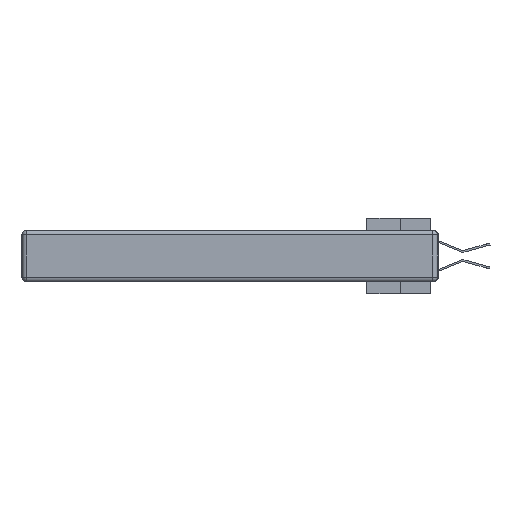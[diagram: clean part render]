
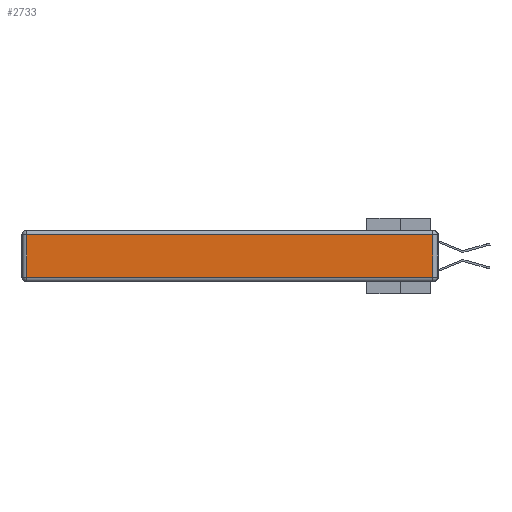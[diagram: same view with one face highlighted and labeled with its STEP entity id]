
A CAD part, left-side view. The second image highlights one B-rep face of the part: STEP entity #2733.
In plain terms, the highlighted planar face has unit normal (-1, 0, 0).
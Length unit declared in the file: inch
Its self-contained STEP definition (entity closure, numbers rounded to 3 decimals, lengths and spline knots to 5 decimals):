
#1680 = DIRECTION ( 'NONE',  ( 0., 0., -1. ) ) ;
#2733 = ADVANCED_FACE ( 'NONE', ( #30033 ), #18449, .T. ) ;
#3042 = CARTESIAN_POINT ( 'NONE',  ( 0., 0.03, -0.343 ) ) ;
#4611 = CARTESIAN_POINT ( 'NONE',  ( 0., 0., -0.343 ) ) ;
#4630 = CARTESIAN_POINT ( 'NONE',  ( 0., 0., -0.313 ) ) ;
#6864 = EDGE_CURVE ( 'NONE', #29253, #25889, #33131, .T. ) ;
#8099 = CARTESIAN_POINT ( 'NONE',  ( 0., 0.03, -0.313 ) ) ;
#9782 = DIRECTION ( 'NONE',  ( 0., -1., 0. ) ) ;
#9823 = VERTEX_POINT ( 'NONE', #8099 ) ;
#10138 = CARTESIAN_POINT ( 'NONE',  ( 0., 2.75, -0.03 ) ) ;
#11704 = AXIS2_PLACEMENT_3D ( 'NONE', #4611, #15663, #29659 ) ;
#13114 = CARTESIAN_POINT ( 'NONE',  ( 0., 2.72, -0.343 ) ) ;
#13416 = VECTOR ( 'NONE', #1680, 39.37008 ) ;
#14109 = EDGE_CURVE ( 'NONE', #9823, #29253, #22403, .T. ) ;
#15663 = DIRECTION ( 'NONE',  ( -1., 0., 0. ) ) ;
#18449 = PLANE ( 'NONE',  #11704 ) ;
#19187 = ORIENTED_EDGE ( 'NONE', *, *, #24821, .T. ) ;
#21542 = ORIENTED_EDGE ( 'NONE', *, *, #6864, .T. ) ;
#22403 = LINE ( 'NONE', #3042, #26266 ) ;
#22550 = VECTOR ( 'NONE', #35528, 39.37008 ) ;
#22754 = CARTESIAN_POINT ( 'NONE',  ( 0., 2.72, -0.03 ) ) ;
#24821 = EDGE_CURVE ( 'NONE', #30087, #9823, #34989, .T. ) ;
#25768 = ORIENTED_EDGE ( 'NONE', *, *, #14109, .T. ) ;
#25889 = VERTEX_POINT ( 'NONE', #22754 ) ;
#25919 = CARTESIAN_POINT ( 'NONE',  ( 0., 0.03, -0.03 ) ) ;
#25964 = CARTESIAN_POINT ( 'NONE',  ( 0., 2.72, -0.313 ) ) ;
#26266 = VECTOR ( 'NONE', #36200, 39.37008 ) ;
#26923 = LINE ( 'NONE', #13114, #13416 ) ;
#26992 = VECTOR ( 'NONE', #9782, 39.37008 ) ;
#28307 = ORIENTED_EDGE ( 'NONE', *, *, #34260, .T. ) ;
#29253 = VERTEX_POINT ( 'NONE', #25919 ) ;
#29659 = DIRECTION ( 'NONE',  ( 0., 0., 1. ) ) ;
#30033 = FACE_OUTER_BOUND ( 'NONE', #30587, .T. ) ;
#30087 = VERTEX_POINT ( 'NONE', #25964 ) ;
#30587 = EDGE_LOOP ( 'NONE', ( #19187, #25768, #21542, #28307 ) ) ;
#33131 = LINE ( 'NONE', #10138, #22550 ) ;
#34260 = EDGE_CURVE ( 'NONE', #25889, #30087, #26923, .T. ) ;
#34989 = LINE ( 'NONE', #4630, #26992 ) ;
#35528 = DIRECTION ( 'NONE',  ( 0., 1., 0. ) ) ;
#36200 = DIRECTION ( 'NONE',  ( 0., 0., 1. ) ) ;
